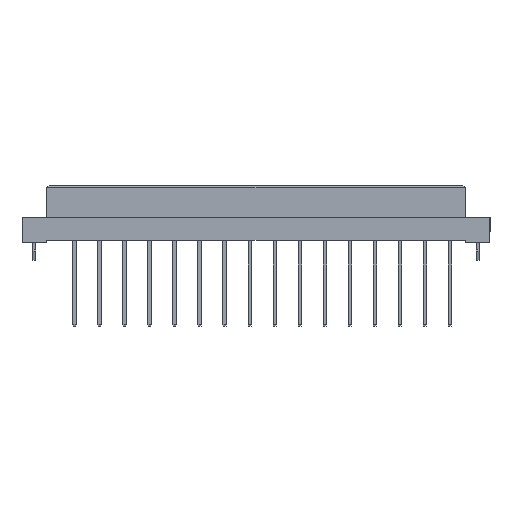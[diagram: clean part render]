
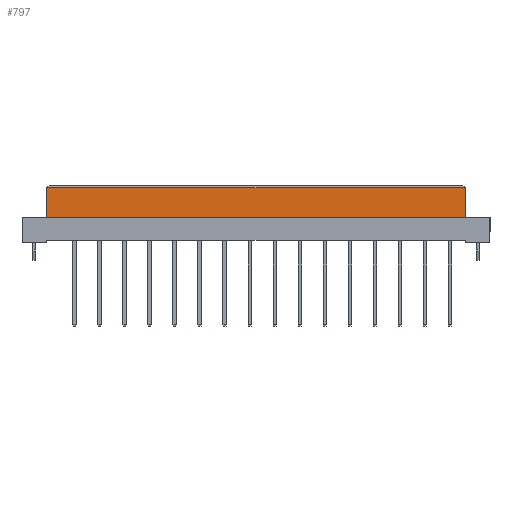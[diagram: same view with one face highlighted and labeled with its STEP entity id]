
A CAD part, top view. The second image highlights one B-rep face of the part: STEP entity #797.
In plain terms, the highlighted planar face has unit normal (0, 0, 1).
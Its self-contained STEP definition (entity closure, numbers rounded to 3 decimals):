
#797 = ADVANCED_FACE ( 'NONE', ( #39215 ), #14365, .T. ) ;
#2985 = CARTESIAN_POINT ( 'NONE',  ( 42.5, -6.4, 4.25 ) ) ;
#5404 = ORIENTED_EDGE ( 'NONE', *, *, #14163, .F. ) ;
#7012 = VERTEX_POINT ( 'NONE', #2985 ) ;
#8603 = AXIS2_PLACEMENT_3D ( 'NONE', #35978, #10959, #32957 ) ;
#9665 = VECTOR ( 'NONE', #17725, 1000. ) ;
#10959 = DIRECTION ( 'NONE',  ( 0., 0., 1. ) ) ;
#12727 = VECTOR ( 'NONE', #30236, 1000. ) ;
#14163 = EDGE_CURVE ( 'NONE', #37272, #26251, #23202, .T. ) ;
#14365 = PLANE ( 'NONE',  #8603 ) ;
#17725 = DIRECTION ( 'NONE',  ( 0., 1., 0. ) ) ;
#18238 = VECTOR ( 'NONE', #32086, 1000. ) ;
#18289 = LINE ( 'NONE', #18494, #12727 ) ;
#18412 = ORIENTED_EDGE ( 'NONE', *, *, #20653, .T. ) ;
#18494 = CARTESIAN_POINT ( 'NONE',  ( 42.5, -6.4, 4.25 ) ) ;
#18806 = EDGE_CURVE ( 'NONE', #37272, #7012, #18289, .T. ) ;
#19259 = CARTESIAN_POINT ( 'NONE',  ( 42.5, -6.4, 4.25 ) ) ;
#19765 = LINE ( 'NONE', #28859, #18238 ) ;
#20653 = EDGE_CURVE ( 'NONE', #7012, #36750, #22291, .T. ) ;
#22291 = LINE ( 'NONE', #19259, #27983 ) ;
#22476 = CARTESIAN_POINT ( 'NONE',  ( -42.5, -6.4, 4.25 ) ) ;
#23202 = LINE ( 'NONE', #32896, #9665 ) ;
#25847 = EDGE_LOOP ( 'NONE', ( #18412, #27170, #5404, #27395 ) ) ;
#26251 = VERTEX_POINT ( 'NONE', #38032 ) ;
#27170 = ORIENTED_EDGE ( 'NONE', *, *, #27216, .T. ) ;
#27216 = EDGE_CURVE ( 'NONE', #36750, #26251, #19765, .T. ) ;
#27395 = ORIENTED_EDGE ( 'NONE', *, *, #18806, .T. ) ;
#27983 = VECTOR ( 'NONE', #34215, 1000. ) ;
#28859 = CARTESIAN_POINT ( 'NONE',  ( -42.5, -0.5, 4.25 ) ) ;
#30236 = DIRECTION ( 'NONE',  ( 1., 0., 0. ) ) ;
#32086 = DIRECTION ( 'NONE',  ( -1., 0., 0. ) ) ;
#32896 = CARTESIAN_POINT ( 'NONE',  ( -42.5, -6.4, 4.25 ) ) ;
#32957 = DIRECTION ( 'NONE',  ( 1., 0., 0. ) ) ;
#33537 = CARTESIAN_POINT ( 'NONE',  ( 42.5, -0.5, 4.25 ) ) ;
#34215 = DIRECTION ( 'NONE',  ( 0., 1., 0. ) ) ;
#35978 = CARTESIAN_POINT ( 'NONE',  ( 42.5, -6.4, 4.25 ) ) ;
#36750 = VERTEX_POINT ( 'NONE', #33537 ) ;
#37272 = VERTEX_POINT ( 'NONE', #22476 ) ;
#38032 = CARTESIAN_POINT ( 'NONE',  ( -42.5, -0.5, 4.25 ) ) ;
#39215 = FACE_OUTER_BOUND ( 'NONE', #25847, .T. ) ;
